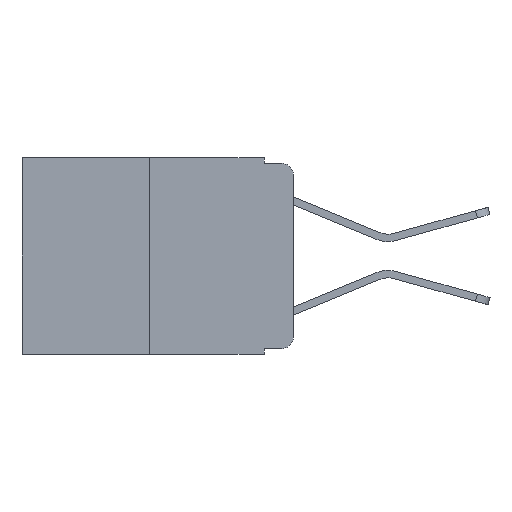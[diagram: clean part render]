
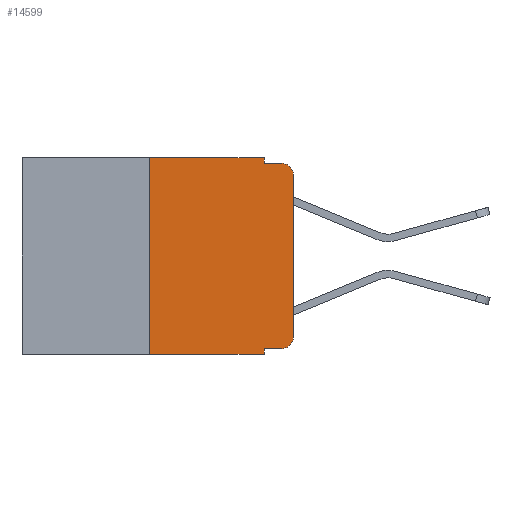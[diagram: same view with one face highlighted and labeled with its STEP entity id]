
A CAD part, left-side view. The second image highlights one B-rep face of the part: STEP entity #14599.
In plain terms, the highlighted planar face has unit normal (-1, 0, 0).
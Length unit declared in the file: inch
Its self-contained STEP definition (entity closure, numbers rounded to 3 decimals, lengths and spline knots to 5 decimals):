
#241 = ORIENTED_EDGE ( 'NONE', *, *, #2933, .T. ) ;
#378 = VECTOR ( 'NONE', #19679, 39.37008 ) ;
#512 = LINE ( 'NONE', #3973, #13303 ) ;
#655 = DIRECTION ( 'NONE',  ( 0., 0., 1. ) ) ;
#691 = PLANE ( 'NONE',  #10948 ) ;
#770 = DIRECTION ( 'NONE',  ( 0., 0., -1. ) ) ;
#1265 = VERTEX_POINT ( 'NONE', #22101 ) ;
#1537 = VECTOR ( 'NONE', #5502, 39.37008 ) ;
#1671 = CARTESIAN_POINT ( 'NONE',  ( 0., 0.25, -0.343 ) ) ;
#1816 = DIRECTION ( 'NONE',  ( 0., 0., -1. ) ) ;
#2141 = EDGE_CURVE ( 'NONE', #1265, #4865, #17777, .T. ) ;
#2320 = ORIENTED_EDGE ( 'NONE', *, *, #2571, .F. ) ;
#2364 = DIRECTION ( 'NONE',  ( 1., 0., 0. ) ) ;
#2376 = DIRECTION ( 'NONE',  ( 0., 0., -1. ) ) ;
#2402 = CARTESIAN_POINT ( 'NONE',  ( 0., 0., 0. ) ) ;
#2436 = CARTESIAN_POINT ( 'NONE',  ( 0., 0.473, 0. ) ) ;
#2571 = EDGE_CURVE ( 'NONE', #9231, #16897, #18295, .T. ) ;
#2933 = EDGE_CURVE ( 'NONE', #5399, #16602, #14464, .T. ) ;
#2941 = CARTESIAN_POINT ( 'NONE',  ( 0., 0.25, 0. ) ) ;
#3296 = ORIENTED_EDGE ( 'NONE', *, *, #3742, .T. ) ;
#3742 = EDGE_CURVE ( 'NONE', #16602, #17342, #13417, .T. ) ;
#3928 = LINE ( 'NONE', #10686, #378 ) ;
#3973 = CARTESIAN_POINT ( 'NONE',  ( 0., 0.051, 0. ) ) ;
#4767 = ORIENTED_EDGE ( 'NONE', *, *, #8906, .F. ) ;
#4865 = VERTEX_POINT ( 'NONE', #11558 ) ;
#5399 = VERTEX_POINT ( 'NONE', #17281 ) ;
#5502 = DIRECTION ( 'NONE',  ( 0., -1., 0. ) ) ;
#5812 = CARTESIAN_POINT ( 'NONE',  ( 0., 0.051, 0. ) ) ;
#6173 = VERTEX_POINT ( 'NONE', #1671 ) ;
#6182 = DIRECTION ( 'NONE',  ( 0., 0., -1. ) ) ;
#6225 = EDGE_CURVE ( 'NONE', #6173, #16897, #19785, .T. ) ;
#6295 = ORIENTED_EDGE ( 'NONE', *, *, #19706, .T. ) ;
#6459 = CARTESIAN_POINT ( 'NONE',  ( 0., 0.473, 0. ) ) ;
#7681 = ORIENTED_EDGE ( 'NONE', *, *, #12473, .F. ) ;
#7962 = EDGE_CURVE ( 'NONE', #9231, #5399, #3928, .T. ) ;
#8299 = ORIENTED_EDGE ( 'NONE', *, *, #17720, .F. ) ;
#8455 = CARTESIAN_POINT ( 'NONE',  ( 0., 0., -0.03 ) ) ;
#8563 = CARTESIAN_POINT ( 'NONE',  ( 0., 0.051, -0.343 ) ) ;
#8708 = CIRCLE ( 'NONE', #20208, 0.02 ) ;
#8805 = FACE_OUTER_BOUND ( 'NONE', #21707, .T. ) ;
#8906 = EDGE_CURVE ( 'NONE', #6173, #1265, #9020, .T. ) ;
#9020 = LINE ( 'NONE', #2941, #20197 ) ;
#9231 = VERTEX_POINT ( 'NONE', #10980 ) ;
#10459 = ORIENTED_EDGE ( 'NONE', *, *, #2141, .F. ) ;
#10570 = CARTESIAN_POINT ( 'NONE',  ( 0., 0.473, -0.343 ) ) ;
#10683 = DIRECTION ( 'NONE',  ( 0., -1., 0. ) ) ;
#10686 = CARTESIAN_POINT ( 'NONE',  ( 0., 0.051, -0.333 ) ) ;
#10948 = AXIS2_PLACEMENT_3D ( 'NONE', #2436, #2364, #770 ) ;
#10980 = CARTESIAN_POINT ( 'NONE',  ( 0., 0.051, -0.333 ) ) ;
#11558 = CARTESIAN_POINT ( 'NONE',  ( 0., 0.051, 0. ) ) ;
#11907 = DIRECTION ( 'NONE',  ( -1., 0., 0. ) ) ;
#12283 = VECTOR ( 'NONE', #2376, 39.37008 ) ;
#12473 = EDGE_CURVE ( 'NONE', #13969, #16941, #18729, .T. ) ;
#12504 = CARTESIAN_POINT ( 'NONE',  ( 0., 0.02, -0.01 ) ) ;
#13303 = VECTOR ( 'NONE', #6182, 39.37008 ) ;
#13417 = LINE ( 'NONE', #2402, #22307 ) ;
#13969 = VERTEX_POINT ( 'NONE', #14580 ) ;
#14464 = CIRCLE ( 'NONE', #15441, 0.02 ) ;
#14509 = VECTOR ( 'NONE', #10683, 39.37008 ) ;
#14580 = CARTESIAN_POINT ( 'NONE',  ( 0., 0.051, -0.01 ) ) ;
#14599 = ADVANCED_FACE ( 'NONE', ( #8805 ), #691, .F. ) ;
#14727 = ORIENTED_EDGE ( 'NONE', *, *, #6225, .T. ) ;
#15417 = DIRECTION ( 'NONE',  ( 0., 0., -1. ) ) ;
#15441 = AXIS2_PLACEMENT_3D ( 'NONE', #15449, #20780, #1816 ) ;
#15449 = CARTESIAN_POINT ( 'NONE',  ( 0., 0.02, -0.313 ) ) ;
#16602 = VERTEX_POINT ( 'NONE', #19906 ) ;
#16897 = VERTEX_POINT ( 'NONE', #8563 ) ;
#16941 = VERTEX_POINT ( 'NONE', #12504 ) ;
#17281 = CARTESIAN_POINT ( 'NONE',  ( 0., 0.02, -0.333 ) ) ;
#17342 = VERTEX_POINT ( 'NONE', #8455 ) ;
#17720 = EDGE_CURVE ( 'NONE', #4865, #13969, #512, .T. ) ;
#17777 = LINE ( 'NONE', #6459, #14509 ) ;
#17835 = CARTESIAN_POINT ( 'NONE',  ( 0., 0.051, -0.01 ) ) ;
#18295 = LINE ( 'NONE', #5812, #12283 ) ;
#18729 = LINE ( 'NONE', #17835, #1537 ) ;
#19546 = DIRECTION ( 'NONE',  ( 0., -1., 0. ) ) ;
#19679 = DIRECTION ( 'NONE',  ( 0., -1., 0. ) ) ;
#19706 = EDGE_CURVE ( 'NONE', #17342, #16941, #8708, .T. ) ;
#19785 = LINE ( 'NONE', #10570, #20878 ) ;
#19906 = CARTESIAN_POINT ( 'NONE',  ( 0., 0., -0.313 ) ) ;
#20197 = VECTOR ( 'NONE', #20358, 39.37008 ) ;
#20208 = AXIS2_PLACEMENT_3D ( 'NONE', #20586, #11907, #15417 ) ;
#20358 = DIRECTION ( 'NONE',  ( 0., 0., 1. ) ) ;
#20586 = CARTESIAN_POINT ( 'NONE',  ( 0., 0.02, -0.03 ) ) ;
#20780 = DIRECTION ( 'NONE',  ( -1., 0., 0. ) ) ;
#20878 = VECTOR ( 'NONE', #19546, 39.37008 ) ;
#21283 = ORIENTED_EDGE ( 'NONE', *, *, #7962, .T. ) ;
#21707 = EDGE_LOOP ( 'NONE', ( #3296, #6295, #7681, #8299, #10459, #4767, #14727, #2320, #21283, #241 ) ) ;
#22101 = CARTESIAN_POINT ( 'NONE',  ( 0., 0.25, 0. ) ) ;
#22307 = VECTOR ( 'NONE', #655, 39.37008 ) ;
